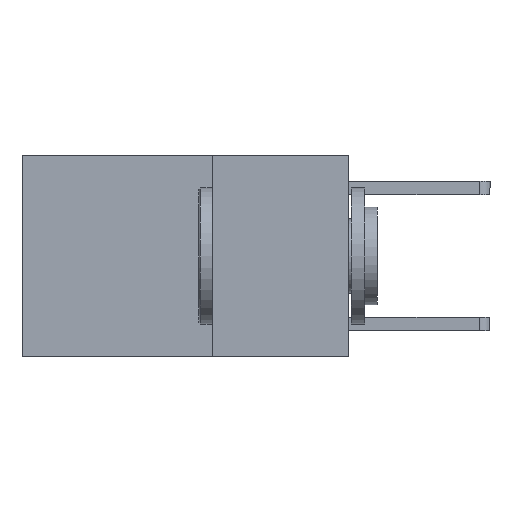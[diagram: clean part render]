
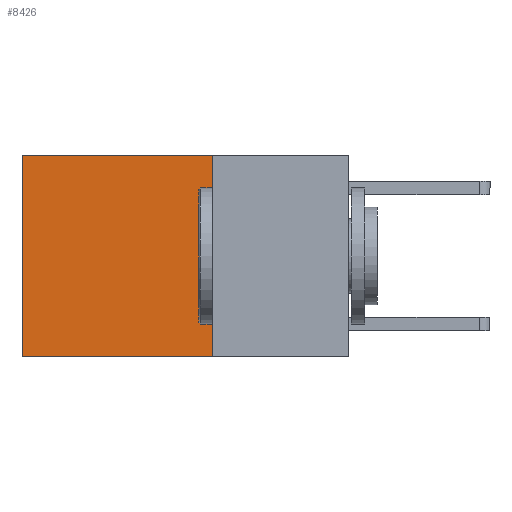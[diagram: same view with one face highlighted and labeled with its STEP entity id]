
A CAD part, left-side view. The second image highlights one B-rep face of the part: STEP entity #8426.
In plain terms, the highlighted planar face has unit normal (-1, 0, 0).
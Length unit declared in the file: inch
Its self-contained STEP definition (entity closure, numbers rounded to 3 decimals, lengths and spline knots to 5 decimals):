
#56 = VERTEX_POINT ( 'NONE', #5924 ) ;
#521 = VERTEX_POINT ( 'NONE', #6296 ) ;
#812 = LINE ( 'NONE', #8337, #5274 ) ;
#841 = AXIS2_PLACEMENT_3D ( 'NONE', #5006, #8063, #6472 ) ;
#1024 = EDGE_LOOP ( 'NONE', ( #3825, #3606, #6560, #2553 ) ) ;
#1908 = DIRECTION ( 'NONE',  ( 0., 0., -1. ) ) ;
#2553 = ORIENTED_EDGE ( 'NONE', *, *, #2755, .T. ) ;
#2601 = LINE ( 'NONE', #9625, #6048 ) ;
#2755 = EDGE_CURVE ( 'NONE', #2907, #521, #8501, .T. ) ;
#2907 = VERTEX_POINT ( 'NONE', #2929 ) ;
#2929 = CARTESIAN_POINT ( 'NONE',  ( 0.2625, 0.25, 0. ) ) ;
#3175 = CARTESIAN_POINT ( 'NONE',  ( 0.2625, 0.25, -0.37 ) ) ;
#3185 = EDGE_CURVE ( 'NONE', #2907, #56, #2601, .T. ) ;
#3361 = VECTOR ( 'NONE', #4812, 39.37008 ) ;
#3606 = ORIENTED_EDGE ( 'NONE', *, *, #5423, .F. ) ;
#3825 = ORIENTED_EDGE ( 'NONE', *, *, #4307, .T. ) ;
#4307 = EDGE_CURVE ( 'NONE', #521, #5992, #812, .T. ) ;
#4812 = DIRECTION ( 'NONE',  ( 0., 1., 0. ) ) ;
#4905 = VECTOR ( 'NONE', #5535, 39.37008 ) ;
#4952 = FACE_OUTER_BOUND ( 'NONE', #1024, .T. ) ;
#5006 = CARTESIAN_POINT ( 'NONE',  ( 0.2625, 0.25, 0. ) ) ;
#5097 = CARTESIAN_POINT ( 'NONE',  ( 0.2625, 0.6, -0.37 ) ) ;
#5274 = VECTOR ( 'NONE', #6948, 39.37008 ) ;
#5423 = EDGE_CURVE ( 'NONE', #56, #5992, #6374, .T. ) ;
#5535 = DIRECTION ( 'NONE',  ( 0., 1., 0. ) ) ;
#5924 = CARTESIAN_POINT ( 'NONE',  ( 0.2625, 0.25, -0.37 ) ) ;
#5992 = VERTEX_POINT ( 'NONE', #5097 ) ;
#6048 = VECTOR ( 'NONE', #1908, 39.37008 ) ;
#6296 = CARTESIAN_POINT ( 'NONE',  ( 0.2625, 0.6, 0. ) ) ;
#6374 = LINE ( 'NONE', #3175, #3361 ) ;
#6472 = DIRECTION ( 'NONE',  ( 0., 0., -1. ) ) ;
#6560 = ORIENTED_EDGE ( 'NONE', *, *, #3185, .F. ) ;
#6948 = DIRECTION ( 'NONE',  ( 0., 0., -1. ) ) ;
#8063 = DIRECTION ( 'NONE',  ( 1., 0., 0. ) ) ;
#8217 = PLANE ( 'NONE',  #841 ) ;
#8337 = CARTESIAN_POINT ( 'NONE',  ( 0.2625, 0.6, 0. ) ) ;
#8426 = ADVANCED_FACE ( 'NONE', ( #4952 ), #8217, .F. ) ;
#8501 = LINE ( 'NONE', #9339, #4905 ) ;
#9339 = CARTESIAN_POINT ( 'NONE',  ( 0.2625, 0.25, 0. ) ) ;
#9625 = CARTESIAN_POINT ( 'NONE',  ( 0.2625, 0.25, 0. ) ) ;
